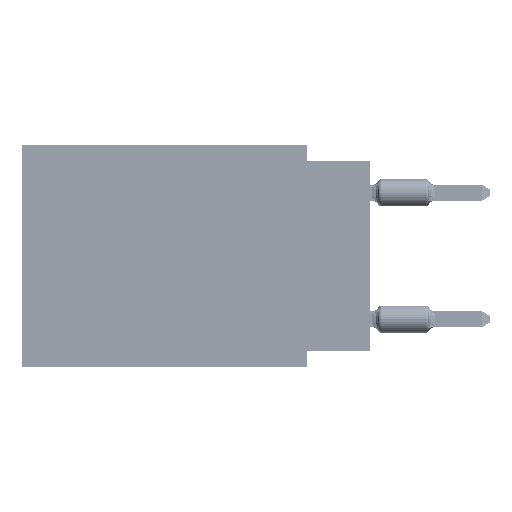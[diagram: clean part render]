
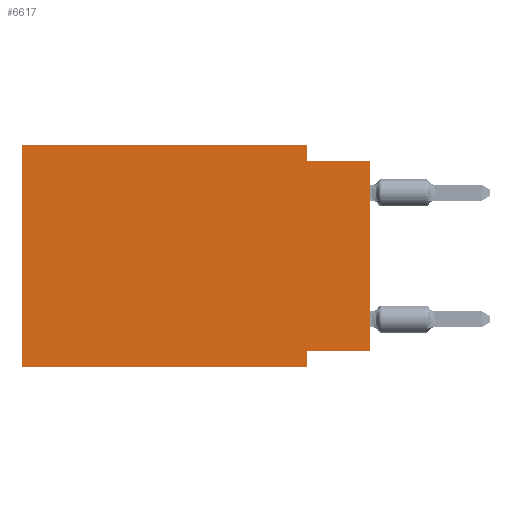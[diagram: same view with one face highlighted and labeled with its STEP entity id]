
A CAD part, left-side view. The second image highlights one B-rep face of the part: STEP entity #6617.
In plain terms, the highlighted planar face has unit normal (-1, 0, 0).
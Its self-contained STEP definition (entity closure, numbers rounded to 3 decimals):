
#1032 = EDGE_LOOP ( 'NONE', ( #44034, #51995, #32005, #24239, #27987, #21120, #26106, #70393 ) ) ;
#3144 = DIRECTION ( 'NONE',  ( 0., 0., 1. ) ) ;
#4110 = EDGE_CURVE ( 'NONE', #46505, #24505, #13597, .T. ) ;
#4886 = CARTESIAN_POINT ( 'NONE',  ( 0., 2.54, -8.89 ) ) ;
#5269 = VECTOR ( 'NONE', #64583, 1000. ) ;
#5693 = VECTOR ( 'NONE', #67767, 1000. ) ;
#6336 = CARTESIAN_POINT ( 'NONE',  ( 0., 2.54, -0.635 ) ) ;
#6617 = ADVANCED_FACE ( 'NONE', ( #9633 ), #22890, .F. ) ;
#8560 = LINE ( 'NONE', #47495, #39945 ) ;
#9480 = VERTEX_POINT ( 'NONE', #39226 ) ;
#9633 = FACE_OUTER_BOUND ( 'NONE', #1032, .T. ) ;
#13597 = LINE ( 'NONE', #67070, #41606 ) ;
#15838 = VECTOR ( 'NONE', #3144, 1000. ) ;
#19989 = VECTOR ( 'NONE', #47775, 1000. ) ;
#21120 = ORIENTED_EDGE ( 'NONE', *, *, #22581, .T. ) ;
#22380 = VECTOR ( 'NONE', #22514, 1000. ) ;
#22514 = DIRECTION ( 'NONE',  ( 0., 0., -1. ) ) ;
#22581 = EDGE_CURVE ( 'NONE', #46505, #27471, #41751, .T. ) ;
#22890 = PLANE ( 'NONE',  #69043 ) ;
#22939 = LINE ( 'NONE', #75149, #22380 ) ;
#24239 = ORIENTED_EDGE ( 'NONE', *, *, #58549, .F. ) ;
#24505 = VERTEX_POINT ( 'NONE', #61209 ) ;
#26106 = ORIENTED_EDGE ( 'NONE', *, *, #74558, .F. ) ;
#27471 = VERTEX_POINT ( 'NONE', #4886 ) ;
#27987 = ORIENTED_EDGE ( 'NONE', *, *, #4110, .F. ) ;
#28490 = LINE ( 'NONE', #41735, #81486 ) ;
#29578 = CARTESIAN_POINT ( 'NONE',  ( 0., 13.97, -8.89 ) ) ;
#30008 = VERTEX_POINT ( 'NONE', #81652 ) ;
#30218 = EDGE_CURVE ( 'NONE', #38578, #9480, #41653, .T. ) ;
#32005 = ORIENTED_EDGE ( 'NONE', *, *, #69991, .F. ) ;
#32049 = CARTESIAN_POINT ( 'NONE',  ( 0., 0., -8.255 ) ) ;
#33544 = EDGE_CURVE ( 'NONE', #71680, #30008, #57727, .T. ) ;
#35491 = DIRECTION ( 'NONE',  ( 0., -1., 0. ) ) ;
#38578 = VERTEX_POINT ( 'NONE', #6336 ) ;
#39226 = CARTESIAN_POINT ( 'NONE',  ( 0., 0., -0.635 ) ) ;
#39945 = VECTOR ( 'NONE', #35491, 1000. ) ;
#41606 = VECTOR ( 'NONE', #65369, 1000. ) ;
#41653 = LINE ( 'NONE', #81451, #5693 ) ;
#41735 = CARTESIAN_POINT ( 'NONE',  ( 0., 2.54, -8.89 ) ) ;
#41751 = LINE ( 'NONE', #55876, #19989 ) ;
#42977 = CARTESIAN_POINT ( 'NONE',  ( 0., 13.97, 0. ) ) ;
#44034 = ORIENTED_EDGE ( 'NONE', *, *, #44402, .T. ) ;
#44402 = EDGE_CURVE ( 'NONE', #71680, #9480, #48501, .T. ) ;
#46505 = VERTEX_POINT ( 'NONE', #29578 ) ;
#47495 = CARTESIAN_POINT ( 'NONE',  ( 0., 13.97, 0. ) ) ;
#47775 = DIRECTION ( 'NONE',  ( 0., -1., 0. ) ) ;
#48184 = DIRECTION ( 'NONE',  ( 0., 0., -1. ) ) ;
#48501 = LINE ( 'NONE', #74588, #15838 ) ;
#49430 = DIRECTION ( 'NONE',  ( 1., 0., 0. ) ) ;
#51995 = ORIENTED_EDGE ( 'NONE', *, *, #30218, .F. ) ;
#53710 = VERTEX_POINT ( 'NONE', #82126 ) ;
#55876 = CARTESIAN_POINT ( 'NONE',  ( 0., 13.97, -8.89 ) ) ;
#57727 = LINE ( 'NONE', #32049, #5269 ) ;
#58549 = EDGE_CURVE ( 'NONE', #24505, #53710, #8560, .T. ) ;
#61209 = CARTESIAN_POINT ( 'NONE',  ( 0., 13.97, 0. ) ) ;
#64583 = DIRECTION ( 'NONE',  ( 0., 1., 0. ) ) ;
#65369 = DIRECTION ( 'NONE',  ( 0., 0., 1. ) ) ;
#67070 = CARTESIAN_POINT ( 'NONE',  ( 0., 13.97, 0. ) ) ;
#67767 = DIRECTION ( 'NONE',  ( 0., -1., 0. ) ) ;
#69043 = AXIS2_PLACEMENT_3D ( 'NONE', #42977, #49430, #75930 ) ;
#69991 = EDGE_CURVE ( 'NONE', #53710, #38578, #22939, .T. ) ;
#70393 = ORIENTED_EDGE ( 'NONE', *, *, #33544, .F. ) ;
#71680 = VERTEX_POINT ( 'NONE', #72920 ) ;
#72920 = CARTESIAN_POINT ( 'NONE',  ( 0., 0., -8.255 ) ) ;
#74558 = EDGE_CURVE ( 'NONE', #30008, #27471, #28490, .T. ) ;
#74588 = CARTESIAN_POINT ( 'NONE',  ( 0., 0., 0. ) ) ;
#75149 = CARTESIAN_POINT ( 'NONE',  ( 0., 2.54, 0. ) ) ;
#75930 = DIRECTION ( 'NONE',  ( 0., 0., -1. ) ) ;
#81451 = CARTESIAN_POINT ( 'NONE',  ( 0., 0., -0.635 ) ) ;
#81486 = VECTOR ( 'NONE', #48184, 1000. ) ;
#81652 = CARTESIAN_POINT ( 'NONE',  ( 0., 2.54, -8.255 ) ) ;
#82126 = CARTESIAN_POINT ( 'NONE',  ( 0., 2.54, 0. ) ) ;
